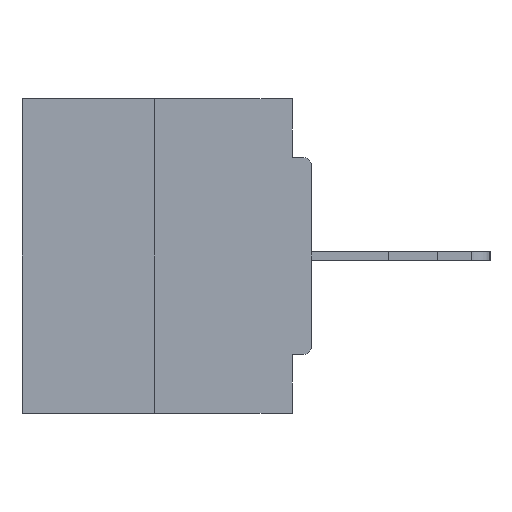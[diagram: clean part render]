
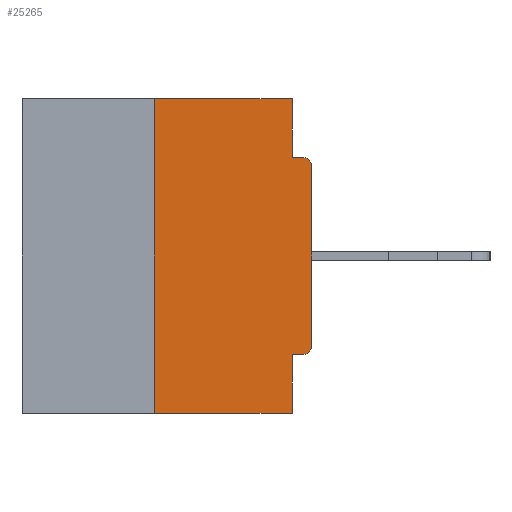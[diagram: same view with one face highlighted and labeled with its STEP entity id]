
A CAD part, left-side view. The second image highlights one B-rep face of the part: STEP entity #25265.
In plain terms, the highlighted planar face has unit normal (-1, 0, 0).
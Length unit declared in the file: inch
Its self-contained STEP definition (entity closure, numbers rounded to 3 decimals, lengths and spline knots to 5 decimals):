
#388 = CARTESIAN_POINT ( 'NONE',  ( 0., 0., -0.1085 ) ) ;
#734 = EDGE_CURVE ( 'NONE', #16926, #11704, #16124, .T. ) ;
#931 = VERTEX_POINT ( 'NONE', #35674 ) ;
#939 = VECTOR ( 'NONE', #24339, 39.37008 ) ;
#2091 = ORIENTED_EDGE ( 'NONE', *, *, #23005, .F. ) ;
#3767 = VECTOR ( 'NONE', #24108, 39.37008 ) ;
#3870 = DIRECTION ( 'NONE',  ( 0., 0., 1. ) ) ;
#3993 = CARTESIAN_POINT ( 'NONE',  ( 0., 0.031, -0.0935 ) ) ;
#4245 = DIRECTION ( 'NONE',  ( -1., 0., 0. ) ) ;
#4815 = VECTOR ( 'NONE', #36479, 39.37008 ) ;
#4889 = VERTEX_POINT ( 'NONE', #22901 ) ;
#4963 = DIRECTION ( 'NONE',  ( 0., 0., -1. ) ) ;
#5019 = ORIENTED_EDGE ( 'NONE', *, *, #34747, .F. ) ;
#6209 = EDGE_CURVE ( 'NONE', #35808, #4889, #34831, .T. ) ;
#6404 = CARTESIAN_POINT ( 'NONE',  ( 0., 0.031, -0.4065 ) ) ;
#6928 = PLANE ( 'NONE',  #30878 ) ;
#7167 = LINE ( 'NONE', #20837, #939 ) ;
#7700 = CARTESIAN_POINT ( 'NONE',  ( 0., 0.015, -0.3915 ) ) ;
#9349 = DIRECTION ( 'NONE',  ( 0., 0., -1. ) ) ;
#9553 = CARTESIAN_POINT ( 'NONE',  ( 0., 0.031, -0.5 ) ) ;
#10272 = VECTOR ( 'NONE', #33284, 39.37008 ) ;
#10396 = EDGE_CURVE ( 'NONE', #35933, #18578, #28761, .T. ) ;
#10760 = CARTESIAN_POINT ( 'NONE',  ( 0., 0.46, -0.5 ) ) ;
#11180 = ORIENTED_EDGE ( 'NONE', *, *, #26229, .F. ) ;
#11639 = VERTEX_POINT ( 'NONE', #6404 ) ;
#11704 = VERTEX_POINT ( 'NONE', #9553 ) ;
#13485 = VERTEX_POINT ( 'NONE', #31684 ) ;
#14602 = ORIENTED_EDGE ( 'NONE', *, *, #10396, .F. ) ;
#14734 = CARTESIAN_POINT ( 'NONE',  ( 0., 0.46, 0. ) ) ;
#15078 = CARTESIAN_POINT ( 'NONE',  ( 0., 0.46, 0. ) ) ;
#15538 = CARTESIAN_POINT ( 'NONE',  ( 0., 0.015, -0.1085 ) ) ;
#15713 = LINE ( 'NONE', #24026, #23202 ) ;
#16124 = LINE ( 'NONE', #10760, #10272 ) ;
#16712 = LINE ( 'NONE', #25220, #4815 ) ;
#16926 = VERTEX_POINT ( 'NONE', #28046 ) ;
#18578 = VERTEX_POINT ( 'NONE', #24499 ) ;
#20444 = DIRECTION ( 'NONE',  ( 0., -1., 0. ) ) ;
#20588 = CARTESIAN_POINT ( 'NONE',  ( 0., 0., -0.4065 ) ) ;
#20773 = LINE ( 'NONE', #20588, #3767 ) ;
#20837 = CARTESIAN_POINT ( 'NONE',  ( 0., 0., 0. ) ) ;
#21268 = VECTOR ( 'NONE', #20444, 39.37008 ) ;
#21434 = AXIS2_PLACEMENT_3D ( 'NONE', #7700, #21929, #29887 ) ;
#21667 = ORIENTED_EDGE ( 'NONE', *, *, #24018, .F. ) ;
#21929 = DIRECTION ( 'NONE',  ( -1., 0., 0. ) ) ;
#22527 = ORIENTED_EDGE ( 'NONE', *, *, #6209, .T. ) ;
#22901 = CARTESIAN_POINT ( 'NONE',  ( 0., 0.015, -0.0935 ) ) ;
#23005 = EDGE_CURVE ( 'NONE', #11639, #11704, #30270, .T. ) ;
#23202 = VECTOR ( 'NONE', #32857, 39.37008 ) ;
#23226 = CIRCLE ( 'NONE', #21434, 0.015 ) ;
#24018 = EDGE_CURVE ( 'NONE', #32258, #4889, #16712, .T. ) ;
#24026 = CARTESIAN_POINT ( 'NONE',  ( 0., 0.031, 0. ) ) ;
#24108 = DIRECTION ( 'NONE',  ( 0., 1., 0. ) ) ;
#24339 = DIRECTION ( 'NONE',  ( 0., 0., 1. ) ) ;
#24499 = CARTESIAN_POINT ( 'NONE',  ( 0., 0.031, 0. ) ) ;
#25220 = CARTESIAN_POINT ( 'NONE',  ( 0., 0., -0.0935 ) ) ;
#25265 = ADVANCED_FACE ( 'NONE', ( #35002 ), #6928, .F. ) ;
#25305 = EDGE_CURVE ( 'NONE', #13485, #11639, #20773, .T. ) ;
#26229 = EDGE_CURVE ( 'NONE', #18578, #32258, #15713, .T. ) ;
#26701 = DIRECTION ( 'NONE',  ( 1., 0., 0. ) ) ;
#26758 = ORIENTED_EDGE ( 'NONE', *, *, #25305, .F. ) ;
#27559 = EDGE_LOOP ( 'NONE', ( #14602, #5019, #34136, #2091, #26758, #27998, #36453, #22527, #21667, #11180 ) ) ;
#27764 = AXIS2_PLACEMENT_3D ( 'NONE', #15538, #4245, #34915 ) ;
#27926 = EDGE_CURVE ( 'NONE', #13485, #931, #23226, .T. ) ;
#27998 = ORIENTED_EDGE ( 'NONE', *, *, #27926, .T. ) ;
#28046 = CARTESIAN_POINT ( 'NONE',  ( 0., 0.25, -0.5 ) ) ;
#28761 = LINE ( 'NONE', #14734, #21268 ) ;
#28814 = CARTESIAN_POINT ( 'NONE',  ( 0., 0.25, 0. ) ) ;
#28817 = VECTOR ( 'NONE', #3870, 39.37008 ) ;
#29887 = DIRECTION ( 'NONE',  ( 0., 0., -1. ) ) ;
#30270 = LINE ( 'NONE', #36195, #32502 ) ;
#30555 = EDGE_CURVE ( 'NONE', #931, #35808, #7167, .T. ) ;
#30878 = AXIS2_PLACEMENT_3D ( 'NONE', #15078, #26701, #9349 ) ;
#31200 = CARTESIAN_POINT ( 'NONE',  ( 0., 0.25, 0. ) ) ;
#31684 = CARTESIAN_POINT ( 'NONE',  ( 0., 0.015, -0.4065 ) ) ;
#32258 = VERTEX_POINT ( 'NONE', #3993 ) ;
#32502 = VECTOR ( 'NONE', #4963, 39.37008 ) ;
#32857 = DIRECTION ( 'NONE',  ( 0., 0., -1. ) ) ;
#33284 = DIRECTION ( 'NONE',  ( 0., -1., 0. ) ) ;
#34136 = ORIENTED_EDGE ( 'NONE', *, *, #734, .T. ) ;
#34355 = LINE ( 'NONE', #28814, #28817 ) ;
#34747 = EDGE_CURVE ( 'NONE', #16926, #35933, #34355, .T. ) ;
#34831 = CIRCLE ( 'NONE', #27764, 0.015 ) ;
#34915 = DIRECTION ( 'NONE',  ( 0., 0., -1. ) ) ;
#35002 = FACE_OUTER_BOUND ( 'NONE', #27559, .T. ) ;
#35674 = CARTESIAN_POINT ( 'NONE',  ( 0., 0., -0.3915 ) ) ;
#35808 = VERTEX_POINT ( 'NONE', #388 ) ;
#35933 = VERTEX_POINT ( 'NONE', #31200 ) ;
#36195 = CARTESIAN_POINT ( 'NONE',  ( 0., 0.031, -0.5 ) ) ;
#36453 = ORIENTED_EDGE ( 'NONE', *, *, #30555, .T. ) ;
#36479 = DIRECTION ( 'NONE',  ( 0., -1., 0. ) ) ;
